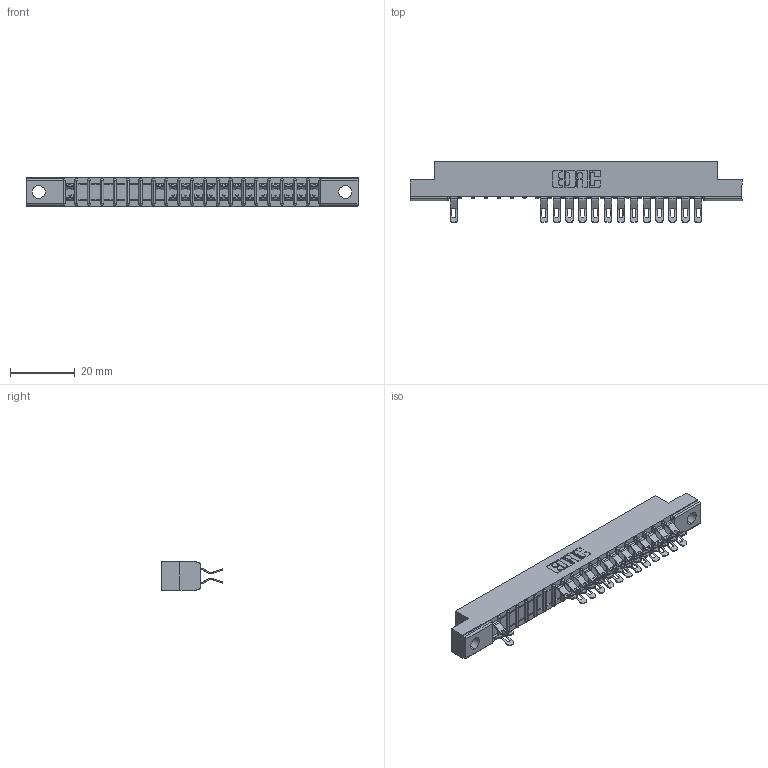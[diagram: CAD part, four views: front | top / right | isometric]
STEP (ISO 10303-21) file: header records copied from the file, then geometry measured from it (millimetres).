
FILE_DESCRIPTION (( 'STEP AP203' ), '1' );
FILE_NAME ('307-040-555-202.STEP', '2018-08-05T15:00:41', ( '' ), ( '' ), 'SwSTEP 2.0', 'SolidWorks 2016', '' );
FILE_SCHEMA (( 'CONFIG_CONTROL_DESIGN' ));
Length unit declared in the file: inch
Products named in the file (3): 307 Part_.128 Dia Mounting Holes; 307-290-001_555; 307-040-555-202
Assembly tree (28 placements, depth 2):
  307-040-555-202
    307 Part_.128 Dia Mounting Holes
    307-290-001_555  x27
Bounding box: 102.26 x 18.75 x 8.71 mm (x, y, z)
Volume: 6513.4 mm3; surface area: 10697.1 mm2
Topology: 28 solids, 28 shells, 1916 faces, 5626 edges, 3656 vertices
Faces by surface type: plane 1066, cylinder 808, sphere 42
Entity records: 20621 total; most frequent: CARTESIAN_POINT 3439, ORIENTED_EDGE 3420, DIRECTION 3372, EDGE_CURVE 1710, VECTOR 1290, LINE 1290, VERTEX_POINT 1108, AXIS2_PLACEMENT_3D 1041
